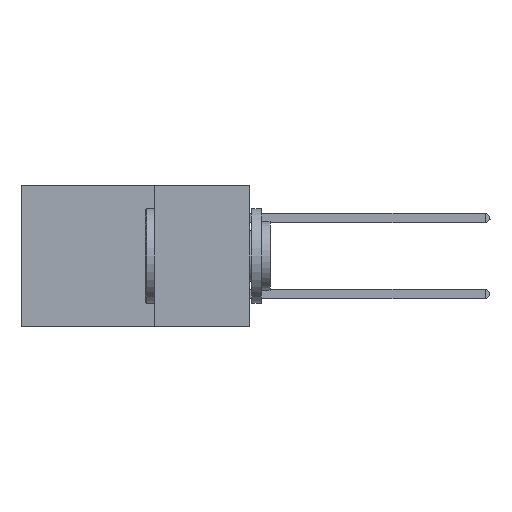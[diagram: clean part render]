
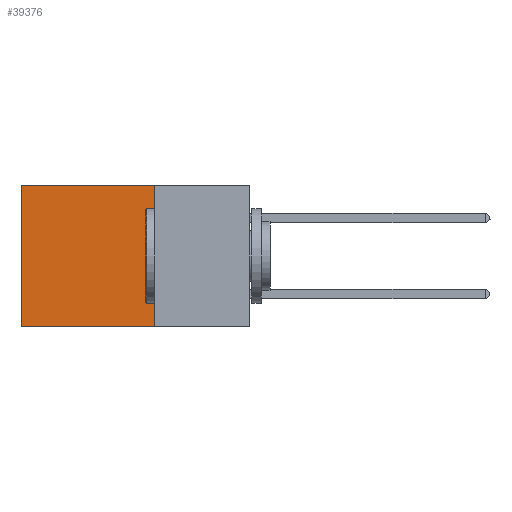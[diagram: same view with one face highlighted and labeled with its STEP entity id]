
A CAD part, left-side view. The second image highlights one B-rep face of the part: STEP entity #39376.
In plain terms, the highlighted planar face has unit normal (-1, 0, 0).
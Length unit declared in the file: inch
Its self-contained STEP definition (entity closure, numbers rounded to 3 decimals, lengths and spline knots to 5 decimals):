
#2548 = CARTESIAN_POINT ( 'NONE',  ( 0.2875, 0.25, 0. ) ) ;
#4596 = EDGE_CURVE ( 'NONE', #16940, #13397, #33320, .T. ) ;
#6219 = ORIENTED_EDGE ( 'NONE', *, *, #4596, .F. ) ;
#9096 = ORIENTED_EDGE ( 'NONE', *, *, #37589, .F. ) ;
#10848 = VECTOR ( 'NONE', #19409, 39.37008 ) ;
#13011 = DIRECTION ( 'NONE',  ( 0., 0., -1. ) ) ;
#13397 = VERTEX_POINT ( 'NONE', #15133 ) ;
#14975 = EDGE_LOOP ( 'NONE', ( #16879, #9096, #6219, #41693 ) ) ;
#15133 = CARTESIAN_POINT ( 'NONE',  ( 0.2875, 0.25, -0.37 ) ) ;
#15942 = DIRECTION ( 'NONE',  ( 0., 1., 0. ) ) ;
#16353 = PLANE ( 'NONE',  #38374 ) ;
#16506 = CARTESIAN_POINT ( 'NONE',  ( 0.2875, 0.25, 0. ) ) ;
#16879 = ORIENTED_EDGE ( 'NONE', *, *, #22627, .T. ) ;
#16940 = VERTEX_POINT ( 'NONE', #23468 ) ;
#17523 = FACE_OUTER_BOUND ( 'NONE', #14975, .T. ) ;
#19409 = DIRECTION ( 'NONE',  ( 0., 1., 0. ) ) ;
#19881 = DIRECTION ( 'NONE',  ( 0., 0., -1. ) ) ;
#21910 = LINE ( 'NONE', #40147, #10848 ) ;
#22627 = EDGE_CURVE ( 'NONE', #37089, #31981, #37246, .T. ) ;
#23468 = CARTESIAN_POINT ( 'NONE',  ( 0.2875, 0.25, 0. ) ) ;
#24144 = DIRECTION ( 'NONE',  ( 0., 0., -1. ) ) ;
#24419 = VECTOR ( 'NONE', #13011, 39.37008 ) ;
#24496 = VECTOR ( 'NONE', #15942, 39.37008 ) ;
#28389 = VECTOR ( 'NONE', #24144, 39.37008 ) ;
#31981 = VERTEX_POINT ( 'NONE', #37497 ) ;
#33320 = LINE ( 'NONE', #43016, #24419 ) ;
#37089 = VERTEX_POINT ( 'NONE', #40470 ) ;
#37246 = LINE ( 'NONE', #40777, #28389 ) ;
#37497 = CARTESIAN_POINT ( 'NONE',  ( 0.2875, 0.6, -0.37 ) ) ;
#37589 = EDGE_CURVE ( 'NONE', #13397, #31981, #21910, .T. ) ;
#38111 = EDGE_CURVE ( 'NONE', #16940, #37089, #42231, .T. ) ;
#38374 = AXIS2_PLACEMENT_3D ( 'NONE', #16506, #39903, #19881 ) ;
#39376 = ADVANCED_FACE ( 'NONE', ( #17523 ), #16353, .F. ) ;
#39903 = DIRECTION ( 'NONE',  ( 1., 0., 0. ) ) ;
#40147 = CARTESIAN_POINT ( 'NONE',  ( 0.2875, 0.25, -0.37 ) ) ;
#40470 = CARTESIAN_POINT ( 'NONE',  ( 0.2875, 0.6, 0. ) ) ;
#40777 = CARTESIAN_POINT ( 'NONE',  ( 0.2875, 0.6, 0. ) ) ;
#41693 = ORIENTED_EDGE ( 'NONE', *, *, #38111, .T. ) ;
#42231 = LINE ( 'NONE', #2548, #24496 ) ;
#43016 = CARTESIAN_POINT ( 'NONE',  ( 0.2875, 0.25, 0. ) ) ;
